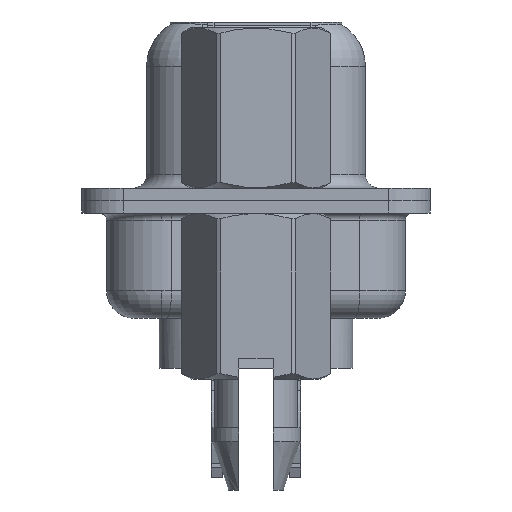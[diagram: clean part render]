
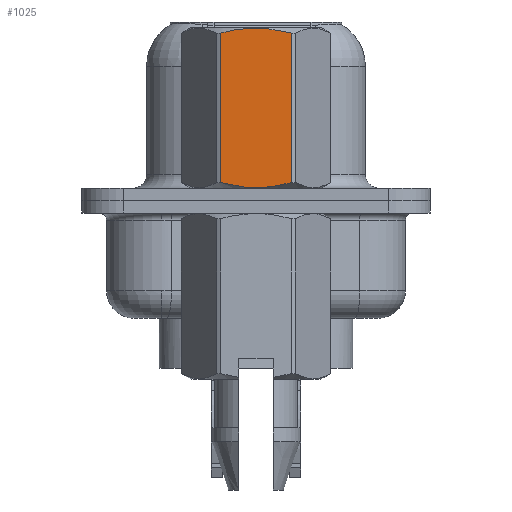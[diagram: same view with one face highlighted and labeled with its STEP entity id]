
A CAD part, left-side view. The second image highlights one B-rep face of the part: STEP entity #1025.
In plain terms, the highlighted planar face has unit normal (-1, 0, 0).
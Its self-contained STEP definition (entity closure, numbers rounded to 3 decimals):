
#291 = DIRECTION ( 'NONE',  ( 0., 0., -1. ) ) ;
#624 = CARTESIAN_POINT ( 'NONE',  ( -2.381, -0.432, 6.215 ) ) ;
#828 = CARTESIAN_POINT ( 'NONE',  ( -2.381, 0.215, 0.468 ) ) ;
#920 = VERTEX_POINT ( 'NONE', #22639 ) ;
#1008 = CARTESIAN_POINT ( 'NONE',  ( -2.381, 1.065, 6.104 ) ) ;
#1025 = ADVANCED_FACE ( 'NONE', ( #4944 ), #24612, .T. ) ;
#1342 = DIRECTION ( 'NONE',  ( 0., 0., 1. ) ) ;
#1441 = EDGE_LOOP ( 'NONE', ( #14686, #23214, #16727, #10526 ) ) ;
#1941 = VERTEX_POINT ( 'NONE', #6744 ) ;
#3124 = VERTEX_POINT ( 'NONE', #17439 ) ;
#4387 = CARTESIAN_POINT ( 'NONE',  ( -2.381, 0.428, 0.485 ) ) ;
#4514 = CARTESIAN_POINT ( 'NONE',  ( -2.381, 1.273, 0.652 ) ) ;
#4944 = FACE_OUTER_BOUND ( 'NONE', #1441, .T. ) ;
#6111 = B_SPLINE_CURVE_WITH_KNOTS ( 'NONE', 3,
 ( #4514, #22335, #18646, #4387, #828, #18777, #14584, #24701, #16424, #6477 ),
 .UNSPECIFIED., .F., .F.,
 ( 4, 2, 2, 2, 4 ),
 ( 0.003, 0.003, 0.004, 0.004, 0.005 ),
 .UNSPECIFIED. ) ;
#6403 = VECTOR ( 'NONE', #291, 1000. ) ;
#6477 = CARTESIAN_POINT ( 'NONE',  ( -2.381, -1.273, 0.652 ) ) ;
#6744 = CARTESIAN_POINT ( 'NONE',  ( -2.381, -1.273, 6.048 ) ) ;
#6932 = EDGE_CURVE ( 'NONE', #18132, #1941, #13137, .T. ) ;
#7133 = EDGE_CURVE ( 'NONE', #920, #3124, #23630, .T. ) ;
#10526 = ORIENTED_EDGE ( 'NONE', *, *, #7133, .T. ) ;
#10936 = EDGE_CURVE ( 'NONE', #3124, #18132, #6111, .T. ) ;
#10962 = CARTESIAN_POINT ( 'NONE',  ( -2.381, 0.428, 6.215 ) ) ;
#12931 = CARTESIAN_POINT ( 'NONE',  ( -2.381, -0.858, 6.15 ) ) ;
#13052 = CARTESIAN_POINT ( 'NONE',  ( -2.381, -0.215, 6.232 ) ) ;
#13137 = LINE ( 'NONE', #13271, #17671 ) ;
#13271 = CARTESIAN_POINT ( 'NONE',  ( -2.381, -1.273, 3.792 ) ) ;
#14584 = CARTESIAN_POINT ( 'NONE',  ( -2.381, -0.432, 0.485 ) ) ;
#14686 = ORIENTED_EDGE ( 'NONE', *, *, #10936, .T. ) ;
#14770 = CARTESIAN_POINT ( 'NONE',  ( -2.381, 1.273, 6.048 ) ) ;
#15046 = CARTESIAN_POINT ( 'NONE',  ( -2.381, -1.273, 0.652 ) ) ;
#16424 = CARTESIAN_POINT ( 'NONE',  ( -2.381, -1.066, 0.596 ) ) ;
#16727 = ORIENTED_EDGE ( 'NONE', *, *, #25043, .T. ) ;
#16746 = CARTESIAN_POINT ( 'NONE',  ( -2.381, 0.853, 6.151 ) ) ;
#17439 = CARTESIAN_POINT ( 'NONE',  ( -2.381, 1.273, 0.652 ) ) ;
#17671 = VECTOR ( 'NONE', #1342, 1000. ) ;
#18018 = B_SPLINE_CURVE_WITH_KNOTS ( 'NONE', 3,
 ( #18577, #25146, #12931, #624, #13052, #18961, #10962, #16746, #1008, #14770 ),
 .UNSPECIFIED., .F., .F.,
 ( 4, 2, 2, 2, 4 ),
 ( 0.001, 0.002, 0.002, 0.003, 0.004 ),
 .UNSPECIFIED. ) ;
#18132 = VERTEX_POINT ( 'NONE', #15046 ) ;
#18577 = CARTESIAN_POINT ( 'NONE',  ( -2.381, -1.273, 6.048 ) ) ;
#18646 = CARTESIAN_POINT ( 'NONE',  ( -2.381, 0.853, 0.549 ) ) ;
#18777 = CARTESIAN_POINT ( 'NONE',  ( -2.381, -0.215, 0.468 ) ) ;
#18961 = CARTESIAN_POINT ( 'NONE',  ( -2.381, 0.215, 6.232 ) ) ;
#20542 = DIRECTION ( 'NONE',  ( -1., 0., 0. ) ) ;
#22186 = CARTESIAN_POINT ( 'NONE',  ( -2.381, 1.273, 3.792 ) ) ;
#22335 = CARTESIAN_POINT ( 'NONE',  ( -2.381, 1.065, 0.596 ) ) ;
#22639 = CARTESIAN_POINT ( 'NONE',  ( -2.381, 1.273, 6.048 ) ) ;
#22768 = DIRECTION ( 'NONE',  ( 0., -1., 0. ) ) ;
#23214 = ORIENTED_EDGE ( 'NONE', *, *, #6932, .T. ) ;
#23630 = LINE ( 'NONE', #22186, #6403 ) ;
#23684 = AXIS2_PLACEMENT_3D ( 'NONE', #24740, #20542, #22768 ) ;
#24612 = PLANE ( 'NONE',  #23684 ) ;
#24701 = CARTESIAN_POINT ( 'NONE',  ( -2.381, -0.858, 0.55 ) ) ;
#24740 = CARTESIAN_POINT ( 'NONE',  ( -2.381, 1.375, -3.75 ) ) ;
#25043 = EDGE_CURVE ( 'NONE', #1941, #920, #18018, .T. ) ;
#25146 = CARTESIAN_POINT ( 'NONE',  ( -2.381, -1.066, 6.104 ) ) ;
